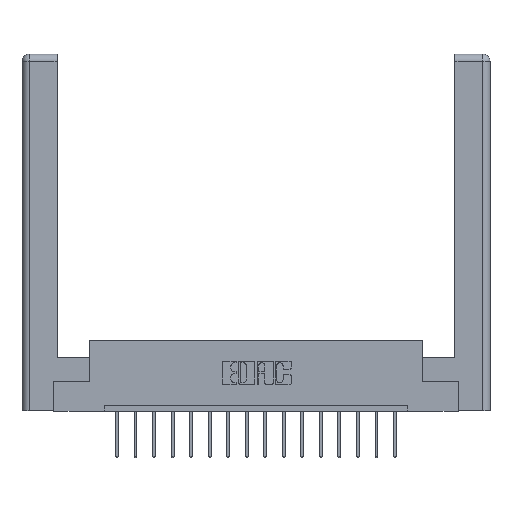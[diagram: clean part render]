
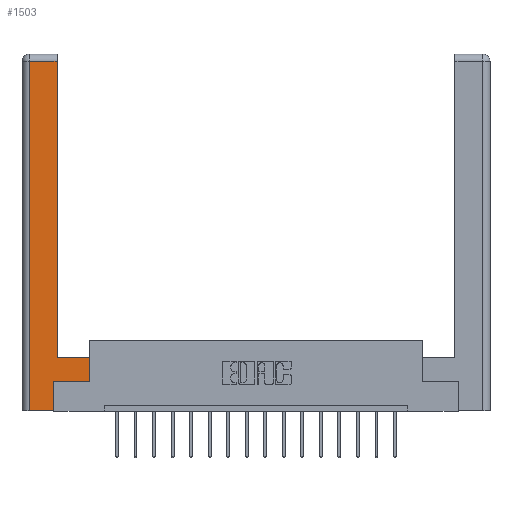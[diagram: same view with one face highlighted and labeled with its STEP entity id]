
A CAD part, top view. The second image highlights one B-rep face of the part: STEP entity #1503.
In plain terms, the highlighted planar face has unit normal (0, 0, 1).
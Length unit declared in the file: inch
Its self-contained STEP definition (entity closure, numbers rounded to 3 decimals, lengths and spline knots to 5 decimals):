
#326 = DIRECTION ( 'NONE',  ( 0., 1., 0. ) ) ;
#427 = EDGE_CURVE ( 'NONE', #3058, #14985, #9737, .T. ) ;
#510 = ORIENTED_EDGE ( 'NONE', *, *, #14041, .T. ) ;
#545 = ORIENTED_EDGE ( 'NONE', *, *, #997, .T. ) ;
#830 = VERTEX_POINT ( 'NONE', #3251 ) ;
#937 = VERTEX_POINT ( 'NONE', #4310 ) ;
#997 = EDGE_CURVE ( 'NONE', #7993, #830, #15112, .T. ) ;
#1503 = ADVANCED_FACE ( 'NONE', ( #4066 ), #12758, .F. ) ;
#1528 = CARTESIAN_POINT ( 'NONE',  ( 0., 0., 0. ) ) ;
#1694 = VECTOR ( 'NONE', #4793, 39.37008 ) ;
#1695 = VECTOR ( 'NONE', #14295, 39.37008 ) ;
#1905 = ORIENTED_EDGE ( 'NONE', *, *, #6516, .T. ) ;
#2225 = VERTEX_POINT ( 'NONE', #7978 ) ;
#2330 = CARTESIAN_POINT ( 'NONE',  ( 0.265, 0.245, 0. ) ) ;
#2442 = ORIENTED_EDGE ( 'NONE', *, *, #13684, .T. ) ;
#2492 = CARTESIAN_POINT ( 'NONE',  ( 0.0615, 0., 0. ) ) ;
#2839 = ORIENTED_EDGE ( 'NONE', *, *, #3049, .T. ) ;
#3049 = EDGE_CURVE ( 'NONE', #830, #937, #7399, .T. ) ;
#3058 = VERTEX_POINT ( 'NONE', #11594 ) ;
#3070 = EDGE_CURVE ( 'NONE', #937, #2225, #17591, .T. ) ;
#3177 = AXIS2_PLACEMENT_3D ( 'NONE', #1528, #14138, #4321 ) ;
#3251 = CARTESIAN_POINT ( 'NONE',  ( 0.565, 0.45, 0. ) ) ;
#3583 = DIRECTION ( 'NONE',  ( 0., -1., 0. ) ) ;
#3820 = CARTESIAN_POINT ( 'NONE',  ( 0.0615, 0., 0. ) ) ;
#3938 = VECTOR ( 'NONE', #326, 39.37008 ) ;
#4066 = FACE_OUTER_BOUND ( 'NONE', #7562, .T. ) ;
#4310 = CARTESIAN_POINT ( 'NONE',  ( 0.295, 0.45, 0. ) ) ;
#4321 = DIRECTION ( 'NONE',  ( -1., 0., 0. ) ) ;
#4362 = VECTOR ( 'NONE', #7343, 39.37008 ) ;
#4662 = CARTESIAN_POINT ( 'NONE',  ( 0.0615, 2.94, 0. ) ) ;
#4793 = DIRECTION ( 'NONE',  ( 0., 1., 0. ) ) ;
#5065 = VERTEX_POINT ( 'NONE', #6331 ) ;
#6331 = CARTESIAN_POINT ( 'NONE',  ( 0.265, 0., 0. ) ) ;
#6516 = EDGE_CURVE ( 'NONE', #6562, #7993, #11411, .T. ) ;
#6562 = VERTEX_POINT ( 'NONE', #2330 ) ;
#7343 = DIRECTION ( 'NONE',  ( -1., 0., 0. ) ) ;
#7399 = LINE ( 'NONE', #16988, #4362 ) ;
#7515 = CARTESIAN_POINT ( 'NONE',  ( 0.565, 0.45, 0. ) ) ;
#7562 = EDGE_LOOP ( 'NONE', ( #8898, #13521, #16475, #510, #2442, #1905, #545, #2839 ) ) ;
#7978 = CARTESIAN_POINT ( 'NONE',  ( 0.295, 2.94, 0. ) ) ;
#7993 = VERTEX_POINT ( 'NONE', #11289 ) ;
#8796 = VECTOR ( 'NONE', #8810, 39.37008 ) ;
#8810 = DIRECTION ( 'NONE',  ( 1., 0., 0. ) ) ;
#8898 = ORIENTED_EDGE ( 'NONE', *, *, #3070, .T. ) ;
#9106 = CARTESIAN_POINT ( 'NONE',  ( 0.565, 0.245, 0. ) ) ;
#9149 = DIRECTION ( 'NONE',  ( 0., 1., 0. ) ) ;
#9452 = LINE ( 'NONE', #17068, #8796 ) ;
#9667 = VECTOR ( 'NONE', #10485, 39.37008 ) ;
#9737 = LINE ( 'NONE', #3820, #17324 ) ;
#10485 = DIRECTION ( 'NONE',  ( 1., 0., 0. ) ) ;
#10546 = LINE ( 'NONE', #14658, #12512 ) ;
#11289 = CARTESIAN_POINT ( 'NONE',  ( 0.565, 0.245, 0. ) ) ;
#11411 = LINE ( 'NONE', #9106, #9667 ) ;
#11594 = CARTESIAN_POINT ( 'NONE',  ( 0.0615, 2.94, 0. ) ) ;
#12512 = VECTOR ( 'NONE', #9149, 39.37008 ) ;
#12758 = PLANE ( 'NONE',  #3177 ) ;
#12821 = CARTESIAN_POINT ( 'NONE',  ( 0.295, 3., 0. ) ) ;
#13521 = ORIENTED_EDGE ( 'NONE', *, *, #17521, .T. ) ;
#13684 = EDGE_CURVE ( 'NONE', #5065, #6562, #10546, .T. ) ;
#14041 = EDGE_CURVE ( 'NONE', #14985, #5065, #9452, .T. ) ;
#14138 = DIRECTION ( 'NONE',  ( 0., 0., -1. ) ) ;
#14295 = DIRECTION ( 'NONE',  ( -1., 0., 0. ) ) ;
#14658 = CARTESIAN_POINT ( 'NONE',  ( 0.265, 0.245, 0. ) ) ;
#14910 = LINE ( 'NONE', #4662, #1695 ) ;
#14985 = VERTEX_POINT ( 'NONE', #2492 ) ;
#15112 = LINE ( 'NONE', #7515, #1694 ) ;
#16475 = ORIENTED_EDGE ( 'NONE', *, *, #427, .T. ) ;
#16988 = CARTESIAN_POINT ( 'NONE',  ( 0.295, 0.45, 0. ) ) ;
#17068 = CARTESIAN_POINT ( 'NONE',  ( 0.265, 0., 0. ) ) ;
#17324 = VECTOR ( 'NONE', #3583, 39.37008 ) ;
#17521 = EDGE_CURVE ( 'NONE', #2225, #3058, #14910, .T. ) ;
#17591 = LINE ( 'NONE', #12821, #3938 ) ;
